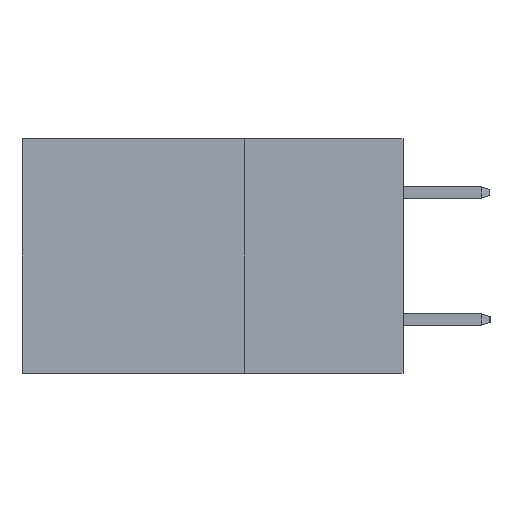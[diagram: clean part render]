
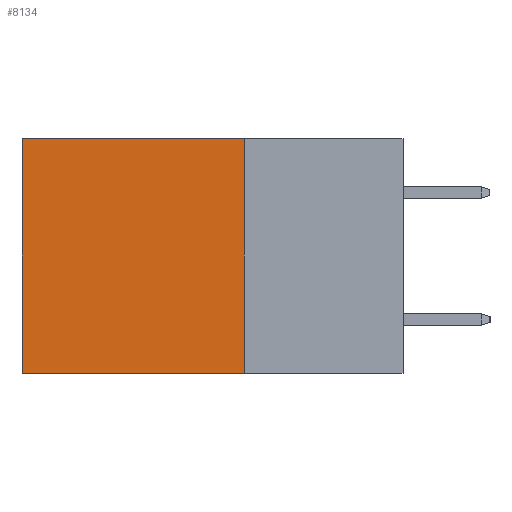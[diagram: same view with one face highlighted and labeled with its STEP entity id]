
A CAD part, left-side view. The second image highlights one B-rep face of the part: STEP entity #8134.
In plain terms, the highlighted planar face has unit normal (-1, 0, 0).
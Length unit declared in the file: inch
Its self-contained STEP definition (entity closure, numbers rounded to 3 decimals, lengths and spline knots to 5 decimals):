
#102 = LINE ( 'NONE', #6491, #7284 ) ;
#141 = CARTESIAN_POINT ( 'NONE',  ( 0.2875, 0.25, 0. ) ) ;
#278 = LINE ( 'NONE', #3083, #8870 ) ;
#857 = ORIENTED_EDGE ( 'NONE', *, *, #2282, .T. ) ;
#1106 = CARTESIAN_POINT ( 'NONE',  ( 0.2875, 0.25, 0. ) ) ;
#1444 = EDGE_LOOP ( 'NONE', ( #857, #8709, #1505, #3921 ) ) ;
#1505 = ORIENTED_EDGE ( 'NONE', *, *, #8045, .F. ) ;
#2225 = CARTESIAN_POINT ( 'NONE',  ( 0.2875, 0.6, 0. ) ) ;
#2242 = CARTESIAN_POINT ( 'NONE',  ( 0.2875, 0.6, -0.37 ) ) ;
#2282 = EDGE_CURVE ( 'NONE', #3719, #4152, #278, .T. ) ;
#2420 = DIRECTION ( 'NONE',  ( 0., 0., -1. ) ) ;
#2591 = VERTEX_POINT ( 'NONE', #141 ) ;
#2753 = LINE ( 'NONE', #2842, #3001 ) ;
#2842 = CARTESIAN_POINT ( 'NONE',  ( 0.2875, 0.25, -0.37 ) ) ;
#3001 = VECTOR ( 'NONE', #4211, 39.37008 ) ;
#3083 = CARTESIAN_POINT ( 'NONE',  ( 0.2875, 0.6, 0. ) ) ;
#3336 = VECTOR ( 'NONE', #6935, 39.37008 ) ;
#3719 = VERTEX_POINT ( 'NONE', #2225 ) ;
#3921 = ORIENTED_EDGE ( 'NONE', *, *, #8949, .T. ) ;
#3995 = DIRECTION ( 'NONE',  ( 1., 0., 0. ) ) ;
#4152 = VERTEX_POINT ( 'NONE', #2242 ) ;
#4211 = DIRECTION ( 'NONE',  ( 0., 1., 0. ) ) ;
#4239 = FACE_OUTER_BOUND ( 'NONE', #1444, .T. ) ;
#4473 = VERTEX_POINT ( 'NONE', #7492 ) ;
#5022 = EDGE_CURVE ( 'NONE', #4473, #4152, #2753, .T. ) ;
#5265 = DIRECTION ( 'NONE',  ( 0., 0., -1. ) ) ;
#5952 = AXIS2_PLACEMENT_3D ( 'NONE', #1106, #3995, #5265 ) ;
#6491 = CARTESIAN_POINT ( 'NONE',  ( 0.2875, 0.25, 0. ) ) ;
#6935 = DIRECTION ( 'NONE',  ( 0., 0., -1. ) ) ;
#7032 = LINE ( 'NONE', #7801, #3336 ) ;
#7091 = DIRECTION ( 'NONE',  ( 0., 1., 0. ) ) ;
#7284 = VECTOR ( 'NONE', #7091, 39.37008 ) ;
#7357 = PLANE ( 'NONE',  #5952 ) ;
#7492 = CARTESIAN_POINT ( 'NONE',  ( 0.2875, 0.25, -0.37 ) ) ;
#7801 = CARTESIAN_POINT ( 'NONE',  ( 0.2875, 0.25, 0. ) ) ;
#8045 = EDGE_CURVE ( 'NONE', #2591, #4473, #7032, .T. ) ;
#8134 = ADVANCED_FACE ( 'NONE', ( #4239 ), #7357, .F. ) ;
#8709 = ORIENTED_EDGE ( 'NONE', *, *, #5022, .F. ) ;
#8870 = VECTOR ( 'NONE', #2420, 39.37008 ) ;
#8949 = EDGE_CURVE ( 'NONE', #2591, #3719, #102, .T. ) ;
